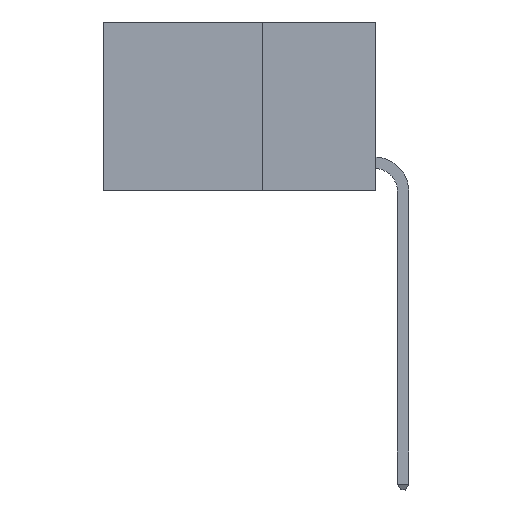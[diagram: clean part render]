
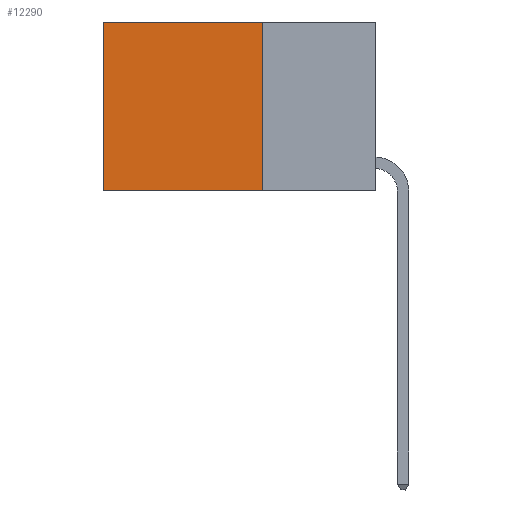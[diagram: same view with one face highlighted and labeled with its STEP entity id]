
A CAD part, left-side view. The second image highlights one B-rep face of the part: STEP entity #12290.
In plain terms, the highlighted planar face has unit normal (-1, 0, 0).
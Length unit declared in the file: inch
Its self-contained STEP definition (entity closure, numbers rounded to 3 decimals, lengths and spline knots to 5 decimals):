
#328 = LINE ( 'NONE', #15246, #20227 ) ;
#568 = LINE ( 'NONE', #13934, #4952 ) ;
#1324 = ORIENTED_EDGE ( 'NONE', *, *, #2011, .T. ) ;
#1477 = CARTESIAN_POINT ( 'NONE',  ( 0.2625, 0.25, 0. ) ) ;
#2011 = EDGE_CURVE ( 'NONE', #17709, #17570, #20429, .T. ) ;
#2280 = VERTEX_POINT ( 'NONE', #14332 ) ;
#3405 = VERTEX_POINT ( 'NONE', #20665 ) ;
#3434 = EDGE_LOOP ( 'NONE', ( #1324, #23152, #8155, #18712 ) ) ;
#4014 = DIRECTION ( 'NONE',  ( 0., 1., 0. ) ) ;
#4450 = EDGE_CURVE ( 'NONE', #2280, #3405, #24066, .T. ) ;
#4952 = VECTOR ( 'NONE', #15816, 39.37008 ) ;
#5082 = CARTESIAN_POINT ( 'NONE',  ( 0.2625, 0.6, -0.37 ) ) ;
#5837 = FACE_OUTER_BOUND ( 'NONE', #3434, .T. ) ;
#6132 = CARTESIAN_POINT ( 'NONE',  ( 0.2625, 0.6, 0. ) ) ;
#6332 = EDGE_CURVE ( 'NONE', #3405, #17570, #568, .T. ) ;
#6785 = CARTESIAN_POINT ( 'NONE',  ( 0.2625, 0.25, 0. ) ) ;
#8155 = ORIENTED_EDGE ( 'NONE', *, *, #4450, .F. ) ;
#8308 = AXIS2_PLACEMENT_3D ( 'NONE', #6785, #8671, #21794 ) ;
#8671 = DIRECTION ( 'NONE',  ( 1., 0., 0. ) ) ;
#9875 = VECTOR ( 'NONE', #21130, 39.37008 ) ;
#12290 = ADVANCED_FACE ( 'NONE', ( #5837 ), #18043, .F. ) ;
#13934 = CARTESIAN_POINT ( 'NONE',  ( 0.2625, 0.25, -0.37 ) ) ;
#14332 = CARTESIAN_POINT ( 'NONE',  ( 0.2625, 0.25, 0. ) ) ;
#14737 = VECTOR ( 'NONE', #16477, 39.37008 ) ;
#15246 = CARTESIAN_POINT ( 'NONE',  ( 0.2625, 0.25, 0. ) ) ;
#15816 = DIRECTION ( 'NONE',  ( 0., 1., 0. ) ) ;
#16477 = DIRECTION ( 'NONE',  ( 0., 0., -1. ) ) ;
#16811 = EDGE_CURVE ( 'NONE', #2280, #17709, #328, .T. ) ;
#17570 = VERTEX_POINT ( 'NONE', #5082 ) ;
#17709 = VERTEX_POINT ( 'NONE', #18603 ) ;
#18043 = PLANE ( 'NONE',  #8308 ) ;
#18603 = CARTESIAN_POINT ( 'NONE',  ( 0.2625, 0.6, 0. ) ) ;
#18712 = ORIENTED_EDGE ( 'NONE', *, *, #16811, .T. ) ;
#20227 = VECTOR ( 'NONE', #4014, 39.37008 ) ;
#20429 = LINE ( 'NONE', #6132, #9875 ) ;
#20665 = CARTESIAN_POINT ( 'NONE',  ( 0.2625, 0.25, -0.37 ) ) ;
#21130 = DIRECTION ( 'NONE',  ( 0., 0., -1. ) ) ;
#21794 = DIRECTION ( 'NONE',  ( 0., 0., -1. ) ) ;
#23152 = ORIENTED_EDGE ( 'NONE', *, *, #6332, .F. ) ;
#24066 = LINE ( 'NONE', #1477, #14737 ) ;
